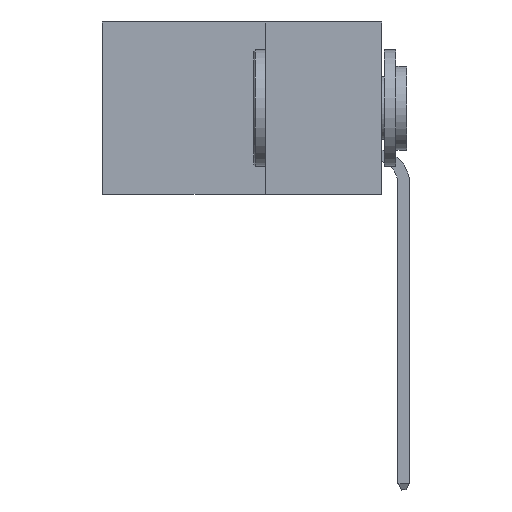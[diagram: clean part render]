
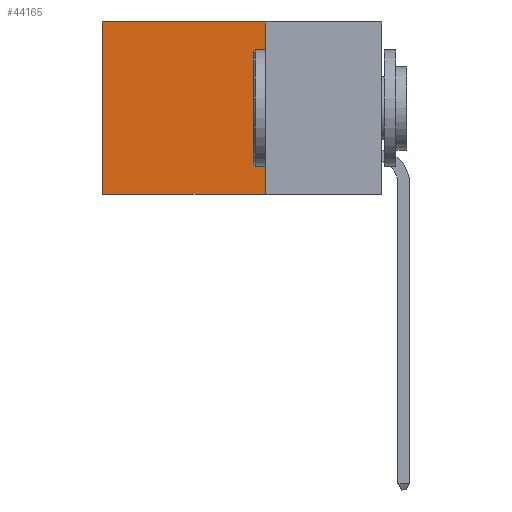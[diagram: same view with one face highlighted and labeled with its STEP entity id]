
A CAD part, left-side view. The second image highlights one B-rep face of the part: STEP entity #44165.
In plain terms, the highlighted planar face has unit normal (-1, 0, 0).
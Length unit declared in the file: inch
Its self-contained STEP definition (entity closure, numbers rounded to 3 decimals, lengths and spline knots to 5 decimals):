
#143 = DIRECTION ( 'NONE',  ( 0., 0., -1. ) ) ;
#476 = CARTESIAN_POINT ( 'NONE',  ( 0.2875, 0.25, -0.37 ) ) ;
#1619 = CARTESIAN_POINT ( 'NONE',  ( 0.2875, 0.25, 0. ) ) ;
#2051 = EDGE_CURVE ( 'NONE', #42467, #23559, #8382, .T. ) ;
#3511 = VERTEX_POINT ( 'NONE', #476 ) ;
#4721 = EDGE_CURVE ( 'NONE', #45018, #42467, #33361, .T. ) ;
#6575 = VECTOR ( 'NONE', #17245, 39.37008 ) ;
#7626 = ORIENTED_EDGE ( 'NONE', *, *, #21607, .F. ) ;
#7851 = AXIS2_PLACEMENT_3D ( 'NONE', #10994, #36652, #143 ) ;
#8382 = LINE ( 'NONE', #40363, #24625 ) ;
#10994 = CARTESIAN_POINT ( 'NONE',  ( 0.2875, 0.25, 0. ) ) ;
#11154 = CARTESIAN_POINT ( 'NONE',  ( 0.2875, 0.6, 0. ) ) ;
#11367 = DIRECTION ( 'NONE',  ( 0., 1., 0. ) ) ;
#15534 = FACE_OUTER_BOUND ( 'NONE', #22195, .T. ) ;
#17245 = DIRECTION ( 'NONE',  ( 0., 1., 0. ) ) ;
#18021 = ORIENTED_EDGE ( 'NONE', *, *, #4721, .T. ) ;
#18582 = VECTOR ( 'NONE', #27019, 39.37008 ) ;
#21607 = EDGE_CURVE ( 'NONE', #45018, #3511, #30049, .T. ) ;
#22195 = EDGE_LOOP ( 'NONE', ( #23925, #22532, #7626, #18021 ) ) ;
#22532 = ORIENTED_EDGE ( 'NONE', *, *, #46042, .F. ) ;
#23559 = VERTEX_POINT ( 'NONE', #31510 ) ;
#23925 = ORIENTED_EDGE ( 'NONE', *, *, #2051, .T. ) ;
#24625 = VECTOR ( 'NONE', #30464, 39.37008 ) ;
#26101 = CARTESIAN_POINT ( 'NONE',  ( 0.2875, 0.25, 0. ) ) ;
#26811 = LINE ( 'NONE', #46754, #42180 ) ;
#27019 = DIRECTION ( 'NONE',  ( 0., 0., -1. ) ) ;
#29207 = PLANE ( 'NONE',  #7851 ) ;
#30049 = LINE ( 'NONE', #1619, #18582 ) ;
#30464 = DIRECTION ( 'NONE',  ( 0., 0., -1. ) ) ;
#31510 = CARTESIAN_POINT ( 'NONE',  ( 0.2875, 0.6, -0.37 ) ) ;
#31966 = CARTESIAN_POINT ( 'NONE',  ( 0.2875, 0.25, 0. ) ) ;
#33361 = LINE ( 'NONE', #31966, #6575 ) ;
#36652 = DIRECTION ( 'NONE',  ( 1., 0., 0. ) ) ;
#40363 = CARTESIAN_POINT ( 'NONE',  ( 0.2875, 0.6, 0. ) ) ;
#42180 = VECTOR ( 'NONE', #11367, 39.37008 ) ;
#42467 = VERTEX_POINT ( 'NONE', #11154 ) ;
#44165 = ADVANCED_FACE ( 'NONE', ( #15534 ), #29207, .F. ) ;
#45018 = VERTEX_POINT ( 'NONE', #26101 ) ;
#46042 = EDGE_CURVE ( 'NONE', #3511, #23559, #26811, .T. ) ;
#46754 = CARTESIAN_POINT ( 'NONE',  ( 0.2875, 0.25, -0.37 ) ) ;
